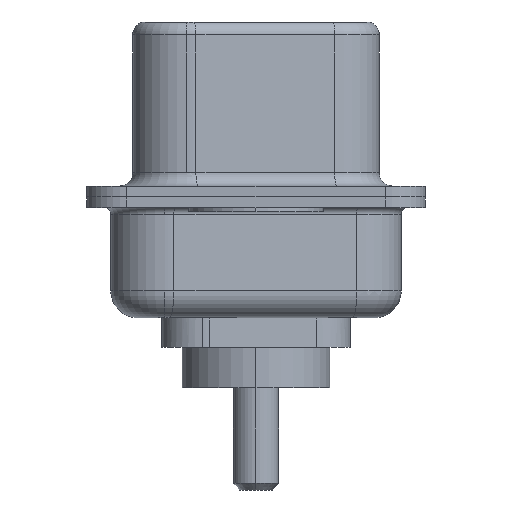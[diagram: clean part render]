
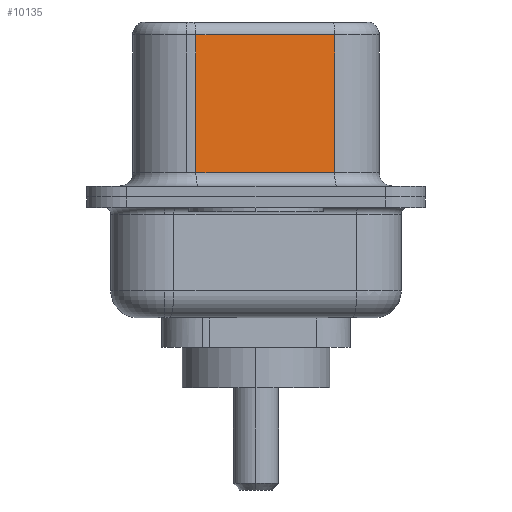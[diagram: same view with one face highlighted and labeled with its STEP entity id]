
A CAD part, left-side view. The second image highlights one B-rep face of the part: STEP entity #10135.
In plain terms, the highlighted planar face has unit normal (-0.985, -0.174, 0).
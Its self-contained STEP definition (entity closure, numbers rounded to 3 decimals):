
#139 = EDGE_CURVE ( 'NONE', #12833, #10574, #2080, .T. ) ;
#454 = DIRECTION ( 'NONE',  ( -0.174, 0.985, 0. ) ) ;
#944 = ORIENTED_EDGE ( 'NONE', *, *, #5539, .F. ) ;
#1463 = VECTOR ( 'NONE', #4182, 1000. ) ;
#1949 = VERTEX_POINT ( 'NONE', #4626 ) ;
#2080 = LINE ( 'NONE', #2738, #12198 ) ;
#2215 = VECTOR ( 'NONE', #6230, 1000. ) ;
#2738 = CARTESIAN_POINT ( 'NONE',  ( 4.565, -2.927, 6.02 ) ) ;
#2771 = FACE_OUTER_BOUND ( 'NONE', #11164, .T. ) ;
#2896 = LINE ( 'NONE', #7316, #12274 ) ;
#3745 = PLANE ( 'NONE',  #10843 ) ;
#4182 = DIRECTION ( 'NONE',  ( 0.174, -0.985, 0. ) ) ;
#4483 = CARTESIAN_POINT ( 'NONE',  ( 3.655, 2.233, 0.9 ) ) ;
#4626 = CARTESIAN_POINT ( 'NONE',  ( 4.565, -2.927, 0.9 ) ) ;
#5136 = CARTESIAN_POINT ( 'NONE',  ( 4.565, -2.927, 6.52 ) ) ;
#5539 = EDGE_CURVE ( 'NONE', #12833, #1949, #12917, .T. ) ;
#5580 = EDGE_CURVE ( 'NONE', #12385, #1949, #10170, .T. ) ;
#5727 = ORIENTED_EDGE ( 'NONE', *, *, #12140, .T. ) ;
#6230 = DIRECTION ( 'NONE',  ( 0., 0., -1. ) ) ;
#7316 = CARTESIAN_POINT ( 'NONE',  ( 3.655, 2.233, 6.52 ) ) ;
#7709 = DIRECTION ( 'NONE',  ( -0.174, 0.985, 0. ) ) ;
#9021 = DIRECTION ( 'NONE',  ( 0., 0., -1. ) ) ;
#9420 = CARTESIAN_POINT ( 'NONE',  ( 4.565, -2.927, 6.02 ) ) ;
#9715 = DIRECTION ( 'NONE',  ( 0.985, 0.174, 0. ) ) ;
#9757 = CARTESIAN_POINT ( 'NONE',  ( 3.655, 2.233, 6.02 ) ) ;
#10135 = ADVANCED_FACE ( 'NONE', ( #2771 ), #3745, .F. ) ;
#10170 = LINE ( 'NONE', #11308, #1463 ) ;
#10574 = VERTEX_POINT ( 'NONE', #9757 ) ;
#10638 = CARTESIAN_POINT ( 'NONE',  ( 4.565, -2.927, 6.52 ) ) ;
#10843 = AXIS2_PLACEMENT_3D ( 'NONE', #5136, #9715, #454 ) ;
#11164 = EDGE_LOOP ( 'NONE', ( #944, #11175, #5727, #12354 ) ) ;
#11175 = ORIENTED_EDGE ( 'NONE', *, *, #139, .T. ) ;
#11308 = CARTESIAN_POINT ( 'NONE',  ( 4.565, -2.927, 0.9 ) ) ;
#12140 = EDGE_CURVE ( 'NONE', #10574, #12385, #2896, .T. ) ;
#12198 = VECTOR ( 'NONE', #7709, 1000. ) ;
#12274 = VECTOR ( 'NONE', #9021, 1000. ) ;
#12354 = ORIENTED_EDGE ( 'NONE', *, *, #5580, .T. ) ;
#12385 = VERTEX_POINT ( 'NONE', #4483 ) ;
#12833 = VERTEX_POINT ( 'NONE', #9420 ) ;
#12917 = LINE ( 'NONE', #10638, #2215 ) ;
